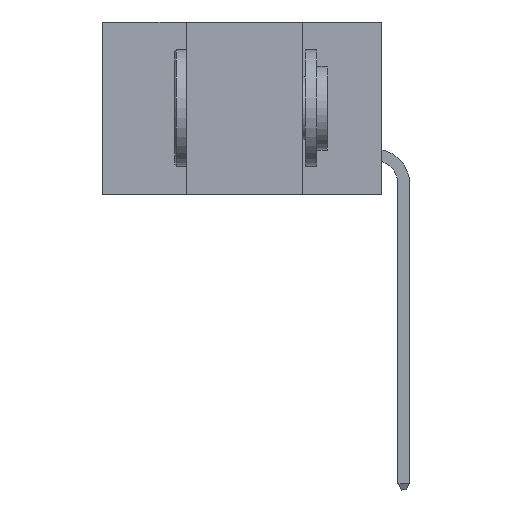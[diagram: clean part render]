
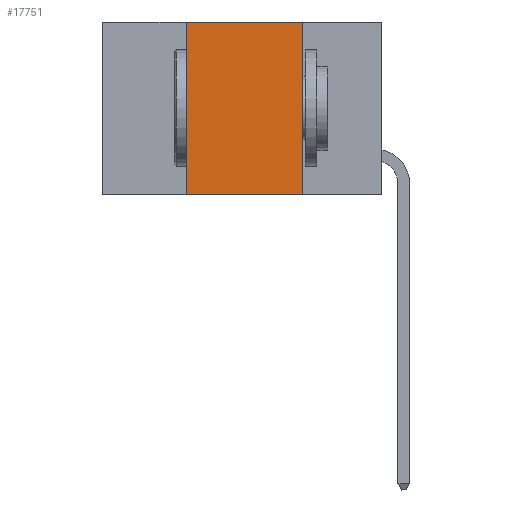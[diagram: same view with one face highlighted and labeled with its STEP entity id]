
A CAD part, left-side view. The second image highlights one B-rep face of the part: STEP entity #17751.
In plain terms, the highlighted planar face has unit normal (-1, 0, 0).
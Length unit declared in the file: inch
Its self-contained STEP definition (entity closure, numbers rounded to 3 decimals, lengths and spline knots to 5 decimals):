
#1591 = DIRECTION ( 'NONE',  ( 0., -1., 0. ) ) ;
#2337 = DIRECTION ( 'NONE',  ( 1., 0., 0. ) ) ;
#4185 = EDGE_CURVE ( 'NONE', #16387, #24002, #14676, .T. ) ;
#5508 = CARTESIAN_POINT ( 'NONE',  ( 0., 0.17, -0.37 ) ) ;
#7968 = EDGE_LOOP ( 'NONE', ( #15286, #15611, #23807, #41119 ) ) ;
#8209 = DIRECTION ( 'NONE',  ( 0., 0., 1. ) ) ;
#8671 = PLANE ( 'NONE',  #18815 ) ;
#10296 = CARTESIAN_POINT ( 'NONE',  ( 0., 0.6, 0. ) ) ;
#13679 = VECTOR ( 'NONE', #8209, 39.37008 ) ;
#14111 = EDGE_CURVE ( 'NONE', #34190, #17730, #25193, .T. ) ;
#14469 = LINE ( 'NONE', #36578, #19958 ) ;
#14676 = LINE ( 'NONE', #23900, #13679 ) ;
#15286 = ORIENTED_EDGE ( 'NONE', *, *, #14111, .F. ) ;
#15611 = ORIENTED_EDGE ( 'NONE', *, *, #32765, .F. ) ;
#16387 = VERTEX_POINT ( 'NONE', #20072 ) ;
#16717 = FACE_OUTER_BOUND ( 'NONE', #7968, .T. ) ;
#16825 = DIRECTION ( 'NONE',  ( 0., -1., 0. ) ) ;
#17730 = VERTEX_POINT ( 'NONE', #5508 ) ;
#17751 = ADVANCED_FACE ( 'NONE', ( #16717 ), #8671, .F. ) ;
#18530 = CARTESIAN_POINT ( 'NONE',  ( 0., 0.17, 0. ) ) ;
#18815 = AXIS2_PLACEMENT_3D ( 'NONE', #36765, #2337, #33829 ) ;
#19958 = VECTOR ( 'NONE', #1591, 39.37008 ) ;
#20072 = CARTESIAN_POINT ( 'NONE',  ( 0., 0.42, -0.37 ) ) ;
#21141 = CARTESIAN_POINT ( 'NONE',  ( 0., 0.17, 0. ) ) ;
#22437 = LINE ( 'NONE', #10296, #33897 ) ;
#23227 = VECTOR ( 'NONE', #40049, 39.37008 ) ;
#23807 = ORIENTED_EDGE ( 'NONE', *, *, #4185, .F. ) ;
#23900 = CARTESIAN_POINT ( 'NONE',  ( 0., 0.42, 0. ) ) ;
#24002 = VERTEX_POINT ( 'NONE', #37574 ) ;
#25193 = LINE ( 'NONE', #21141, #23227 ) ;
#32765 = EDGE_CURVE ( 'NONE', #24002, #34190, #22437, .T. ) ;
#32931 = EDGE_CURVE ( 'NONE', #16387, #17730, #14469, .T. ) ;
#33829 = DIRECTION ( 'NONE',  ( 0., 0., -1. ) ) ;
#33897 = VECTOR ( 'NONE', #16825, 39.37008 ) ;
#34190 = VERTEX_POINT ( 'NONE', #18530 ) ;
#36578 = CARTESIAN_POINT ( 'NONE',  ( 0., 0.6, -0.37 ) ) ;
#36765 = CARTESIAN_POINT ( 'NONE',  ( 0., 0.6, 0. ) ) ;
#37574 = CARTESIAN_POINT ( 'NONE',  ( 0., 0.42, 0. ) ) ;
#40049 = DIRECTION ( 'NONE',  ( 0., 0., -1. ) ) ;
#41119 = ORIENTED_EDGE ( 'NONE', *, *, #32931, .T. ) ;
